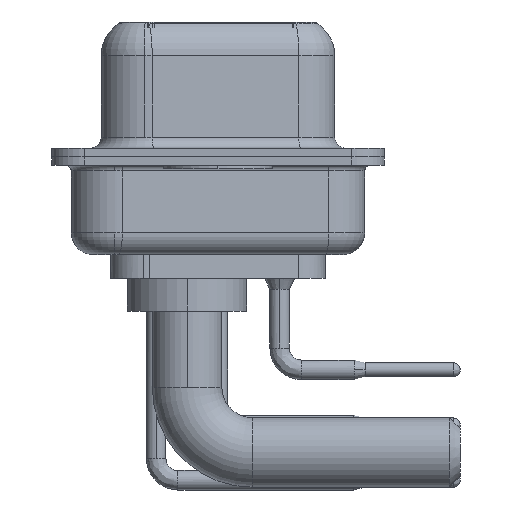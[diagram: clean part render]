
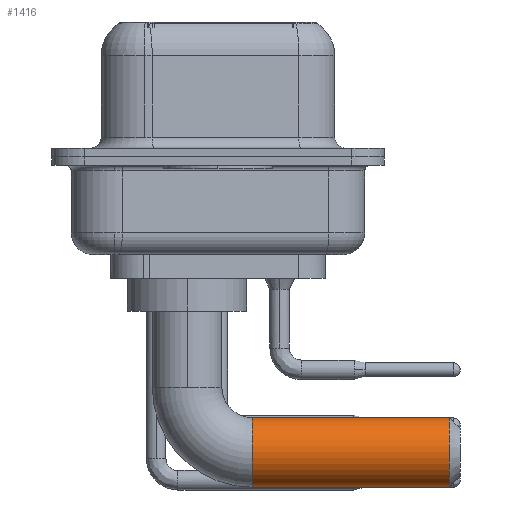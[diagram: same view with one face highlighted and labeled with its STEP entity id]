
A CAD part, left-side view. The second image highlights one B-rep face of the part: STEP entity #1416.
In plain terms, the highlighted cylindrical face has radius 1.6 mm (diameter 3.2 mm), a partial arc.
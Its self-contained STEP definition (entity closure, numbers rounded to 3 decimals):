
#176 = LINE ( 'NONE', #16766, #15896 ) ;
#853 = VERTEX_POINT ( 'NONE', #13702 ) ;
#1114 = VERTEX_POINT ( 'NONE', #15891 ) ;
#1416 = ADVANCED_FACE ( 'NONE', ( #3632 ), #1523, .T. ) ;
#1523 = CYLINDRICAL_SURFACE ( 'NONE', #12204, 1.6 ) ;
#1673 = DIRECTION ( 'NONE',  ( 0., 0., -1. ) ) ;
#1699 = EDGE_CURVE ( 'NONE', #20146, #853, #19751, .T. ) ;
#1886 = CARTESIAN_POINT ( 'NONE',  ( 0., -3., -8.1 ) ) ;
#3632 = FACE_OUTER_BOUND ( 'NONE', #6730, .T. ) ;
#4069 = ORIENTED_EDGE ( 'NONE', *, *, #27487, .F. ) ;
#6193 = DIRECTION ( 'NONE',  ( 0., -1., 0. ) ) ;
#6496 = LINE ( 'NONE', #1886, #12911 ) ;
#6730 = EDGE_LOOP ( 'NONE', ( #4069, #9342, #15961, #22358 ) ) ;
#6767 = DIRECTION ( 'NONE',  ( 0., -1., 0. ) ) ;
#6823 = DIRECTION ( 'NONE',  ( -1., 0., 0. ) ) ;
#7377 = DIRECTION ( 'NONE',  ( 0., -1., 0. ) ) ;
#7817 = VERTEX_POINT ( 'NONE', #26820 ) ;
#9342 = ORIENTED_EDGE ( 'NONE', *, *, #1699, .T. ) ;
#10043 = CARTESIAN_POINT ( 'NONE',  ( 0., -3., -6.5 ) ) ;
#12204 = AXIS2_PLACEMENT_3D ( 'NONE', #10043, #18547, #1673 ) ;
#12911 = VECTOR ( 'NONE', #6767, 1000. ) ;
#13702 = CARTESIAN_POINT ( 'NONE',  ( 0., -3., -8.1 ) ) ;
#14192 = CIRCLE ( 'NONE', #26675, 1.6 ) ;
#15541 = EDGE_CURVE ( 'NONE', #7817, #1114, #14192, .T. ) ;
#15891 = CARTESIAN_POINT ( 'NONE',  ( 0., -12.07, -4.9 ) ) ;
#15896 = VECTOR ( 'NONE', #6193, 1000. ) ;
#15961 = ORIENTED_EDGE ( 'NONE', *, *, #16999, .T. ) ;
#16766 = CARTESIAN_POINT ( 'NONE',  ( 0., -3., -4.9 ) ) ;
#16999 = EDGE_CURVE ( 'NONE', #853, #7817, #6496, .T. ) ;
#17523 = AXIS2_PLACEMENT_3D ( 'NONE', #26456, #7377, #6823 ) ;
#17583 = DIRECTION ( 'NONE',  ( 0., 1., 0. ) ) ;
#18547 = DIRECTION ( 'NONE',  ( 0., -1., 0. ) ) ;
#19751 = CIRCLE ( 'NONE', #17523, 1.6 ) ;
#20146 = VERTEX_POINT ( 'NONE', #27296 ) ;
#21350 = DIRECTION ( 'NONE',  ( 0., 0., -1. ) ) ;
#21634 = CARTESIAN_POINT ( 'NONE',  ( 0., -12.07, -6.5 ) ) ;
#22358 = ORIENTED_EDGE ( 'NONE', *, *, #15541, .T. ) ;
#26456 = CARTESIAN_POINT ( 'NONE',  ( 0., -3., -6.5 ) ) ;
#26675 = AXIS2_PLACEMENT_3D ( 'NONE', #21634, #17583, #21350 ) ;
#26820 = CARTESIAN_POINT ( 'NONE',  ( 0., -12.07, -8.1 ) ) ;
#27296 = CARTESIAN_POINT ( 'NONE',  ( 0., -3., -4.9 ) ) ;
#27487 = EDGE_CURVE ( 'NONE', #20146, #1114, #176, .T. ) ;
